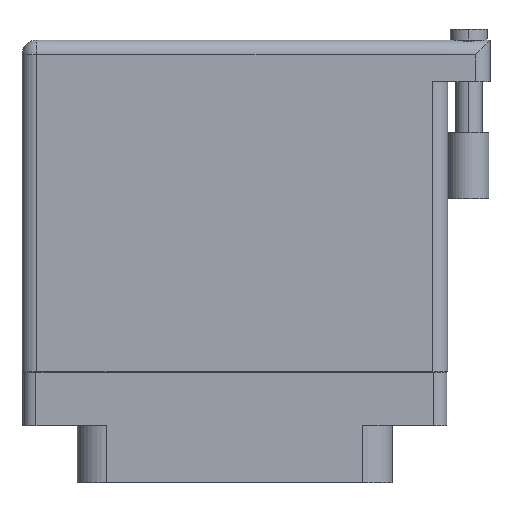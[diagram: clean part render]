
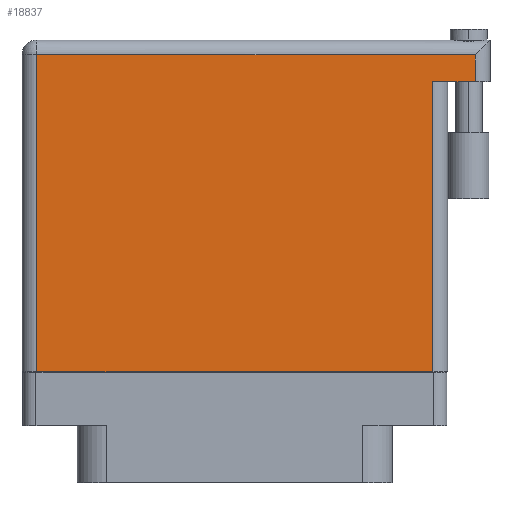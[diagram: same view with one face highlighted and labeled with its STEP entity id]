
A CAD part, front view. The second image highlights one B-rep face of the part: STEP entity #18837.
In plain terms, the highlighted face is planar.
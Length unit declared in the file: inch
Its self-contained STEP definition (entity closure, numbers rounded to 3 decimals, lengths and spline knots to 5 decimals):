
#721 = CARTESIAN_POINT ( 'NONE',  ( -0.934, -0.1, 0.4495 ) ) ;
#752 = VERTEX_POINT ( 'NONE', #3483 ) ;
#1187 = EDGE_CURVE ( 'NONE', #27850, #13976, #4222, .T. ) ;
#1511 = DIRECTION ( 'NONE',  ( -1., 0., 0. ) ) ;
#2097 = VECTOR ( 'NONE', #38703, 39.37008 ) ;
#2748 = PLANE ( 'NONE',  #38306 ) ;
#3483 = CARTESIAN_POINT ( 'NONE',  ( 0.934, -0.1, 0.4495 ) ) ;
#3760 = VECTOR ( 'NONE', #7095, 39.37008 ) ;
#3784 = DIRECTION ( 'NONE',  ( 0., 1., 0. ) ) ;
#4222 = LINE ( 'NONE', #4430, #3760 ) ;
#4309 = FACE_OUTER_BOUND ( 'NONE', #25064, .T. ) ;
#4430 = CARTESIAN_POINT ( 'NONE',  ( 1.134, 1.466, 0.4495 ) ) ;
#5834 = DIRECTION ( 'NONE',  ( 0., 0., -1. ) ) ;
#5853 = VERTEX_POINT ( 'NONE', #721 ) ;
#6004 = ORIENTED_EDGE ( 'NONE', *, *, #1187, .T. ) ;
#7095 = DIRECTION ( 'NONE',  ( 0., 1., 0. ) ) ;
#7189 = CARTESIAN_POINT ( 'NONE',  ( 0.934, 1.269, 0.4495 ) ) ;
#11415 = VERTEX_POINT ( 'NONE', #34951 ) ;
#11715 = DIRECTION ( 'NONE',  ( 1., 0., 0. ) ) ;
#13976 = VERTEX_POINT ( 'NONE', #39100 ) ;
#14103 = CARTESIAN_POINT ( 'NONE',  ( -0.934, -0.1, 0.4495 ) ) ;
#16248 = EDGE_CURVE ( 'NONE', #11415, #5853, #25560, .T. ) ;
#16390 = ORIENTED_EDGE ( 'NONE', *, *, #16248, .T. ) ;
#18837 = ADVANCED_FACE ( 'NONE', ( #4309 ), #2748, .F. ) ;
#21313 = DIRECTION ( 'NONE',  ( -1., 0., 0. ) ) ;
#21669 = DIRECTION ( 'NONE',  ( -1., 0., 0. ) ) ;
#22030 = VECTOR ( 'NONE', #1511, 39.37008 ) ;
#23532 = LINE ( 'NONE', #34317, #38951 ) ;
#25064 = EDGE_LOOP ( 'NONE', ( #28549, #25505, #35573, #6004, #33932, #16390 ) ) ;
#25505 = ORIENTED_EDGE ( 'NONE', *, *, #38986, .T. ) ;
#25560 = LINE ( 'NONE', #14103, #2097 ) ;
#26143 = LINE ( 'NONE', #29961, #29515 ) ;
#26430 = VECTOR ( 'NONE', #3784, 39.37008 ) ;
#27850 = VERTEX_POINT ( 'NONE', #36491 ) ;
#28280 = CARTESIAN_POINT ( 'NONE',  ( 0.934, 1.269, 0.4495 ) ) ;
#28549 = ORIENTED_EDGE ( 'NONE', *, *, #29361, .T. ) ;
#29068 = VERTEX_POINT ( 'NONE', #7189 ) ;
#29361 = EDGE_CURVE ( 'NONE', #5853, #752, #26143, .T. ) ;
#29515 = VECTOR ( 'NONE', #11715, 39.37008 ) ;
#29961 = CARTESIAN_POINT ( 'NONE',  ( -1.004, -0.1, 0.4495 ) ) ;
#33932 = ORIENTED_EDGE ( 'NONE', *, *, #34803, .T. ) ;
#34317 = CARTESIAN_POINT ( 'NONE',  ( -1.004, 1.396, 0.4495 ) ) ;
#34803 = EDGE_CURVE ( 'NONE', #13976, #11415, #23532, .T. ) ;
#34951 = CARTESIAN_POINT ( 'NONE',  ( -0.934, 1.396, 0.4495 ) ) ;
#35398 = EDGE_CURVE ( 'NONE', #27850, #29068, #35997, .T. ) ;
#35573 = ORIENTED_EDGE ( 'NONE', *, *, #35398, .F. ) ;
#35997 = LINE ( 'NONE', #38095, #22030 ) ;
#36491 = CARTESIAN_POINT ( 'NONE',  ( 1.134, 1.269, 0.4495 ) ) ;
#37529 = LINE ( 'NONE', #28280, #26430 ) ;
#38095 = CARTESIAN_POINT ( 'NONE',  ( 1.204, 1.269, 0.4495 ) ) ;
#38306 = AXIS2_PLACEMENT_3D ( 'NONE', #39783, #5834, #21313 ) ;
#38703 = DIRECTION ( 'NONE',  ( 0., -1., 0. ) ) ;
#38951 = VECTOR ( 'NONE', #21669, 39.37008 ) ;
#38986 = EDGE_CURVE ( 'NONE', #752, #29068, #37529, .T. ) ;
#39100 = CARTESIAN_POINT ( 'NONE',  ( 1.134, 1.396, 0.4495 ) ) ;
#39783 = CARTESIAN_POINT ( 'NONE',  ( -1.004, 1.466, 0.4495 ) ) ;
